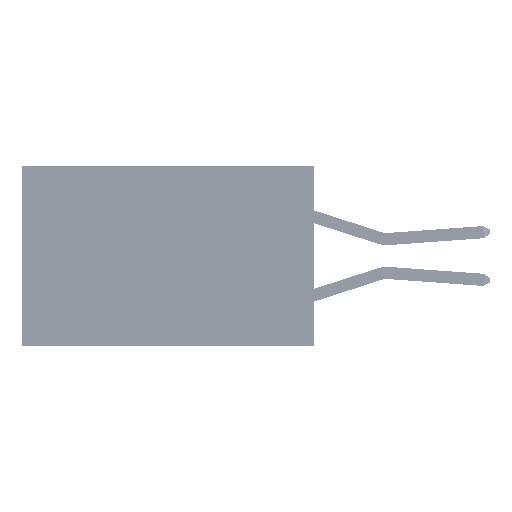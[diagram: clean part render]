
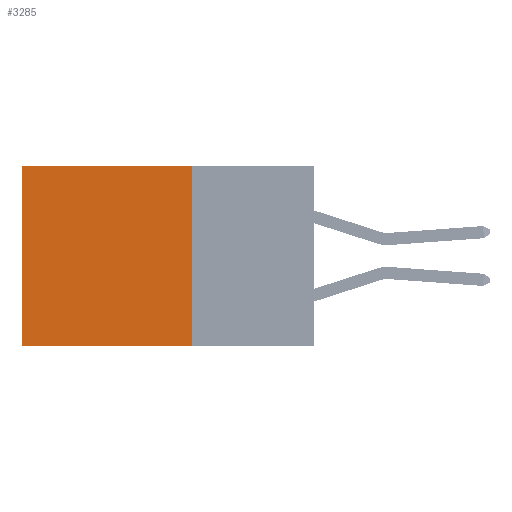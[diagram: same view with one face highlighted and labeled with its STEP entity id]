
A CAD part, left-side view. The second image highlights one B-rep face of the part: STEP entity #3285.
In plain terms, the highlighted planar face has unit normal (-1, 0, 0).
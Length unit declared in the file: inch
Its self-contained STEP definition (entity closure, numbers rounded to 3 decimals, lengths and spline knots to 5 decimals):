
#3029 = DIRECTION ( 'NONE',  ( 0., 0., -1. ) ) ;
#3264 = DIRECTION ( 'NONE',  ( 0., 0., -1. ) ) ;
#3285 = ADVANCED_FACE ( 'NONE', ( #26537 ), #45594, .F. ) ;
#4082 = CARTESIAN_POINT ( 'NONE',  ( 0.2875, 0.6, 0. ) ) ;
#5097 = EDGE_LOOP ( 'NONE', ( #41890, #22316, #21248, #32112 ) ) ;
#6092 = LINE ( 'NONE', #32702, #40562 ) ;
#8601 = EDGE_CURVE ( 'NONE', #42347, #35411, #6092, .T. ) ;
#11349 = EDGE_CURVE ( 'NONE', #30281, #12257, #35997, .T. ) ;
#12257 = VERTEX_POINT ( 'NONE', #42336 ) ;
#12321 = DIRECTION ( 'NONE',  ( 0., 1., 0. ) ) ;
#15935 = VECTOR ( 'NONE', #3029, 39.37008 ) ;
#16419 = EDGE_CURVE ( 'NONE', #42347, #30281, #29291, .T. ) ;
#17265 = DIRECTION ( 'NONE',  ( 1., 0., 0. ) ) ;
#18096 = DIRECTION ( 'NONE',  ( 0., 1., 0. ) ) ;
#20285 = LINE ( 'NONE', #43575, #38691 ) ;
#21248 = ORIENTED_EDGE ( 'NONE', *, *, #8601, .F. ) ;
#22316 = ORIENTED_EDGE ( 'NONE', *, *, #27021, .F. ) ;
#25839 = AXIS2_PLACEMENT_3D ( 'NONE', #35321, #17265, #3264 ) ;
#26537 = FACE_OUTER_BOUND ( 'NONE', #5097, .T. ) ;
#27021 = EDGE_CURVE ( 'NONE', #35411, #12257, #20285, .T. ) ;
#29291 = LINE ( 'NONE', #40447, #41547 ) ;
#30281 = VERTEX_POINT ( 'NONE', #4082 ) ;
#32112 = ORIENTED_EDGE ( 'NONE', *, *, #16419, .T. ) ;
#32702 = CARTESIAN_POINT ( 'NONE',  ( 0.2875, 0.25, 0. ) ) ;
#35058 = CARTESIAN_POINT ( 'NONE',  ( 0.2875, 0.6, 0. ) ) ;
#35321 = CARTESIAN_POINT ( 'NONE',  ( 0.2875, 0.25, 0. ) ) ;
#35411 = VERTEX_POINT ( 'NONE', #44801 ) ;
#35997 = LINE ( 'NONE', #35058, #15935 ) ;
#37927 = CARTESIAN_POINT ( 'NONE',  ( 0.2875, 0.25, 0. ) ) ;
#38688 = DIRECTION ( 'NONE',  ( 0., 0., -1. ) ) ;
#38691 = VECTOR ( 'NONE', #18096, 39.37008 ) ;
#40447 = CARTESIAN_POINT ( 'NONE',  ( 0.2875, 0.25, 0. ) ) ;
#40562 = VECTOR ( 'NONE', #38688, 39.37008 ) ;
#41547 = VECTOR ( 'NONE', #12321, 39.37008 ) ;
#41890 = ORIENTED_EDGE ( 'NONE', *, *, #11349, .T. ) ;
#42336 = CARTESIAN_POINT ( 'NONE',  ( 0.2875, 0.6, -0.37 ) ) ;
#42347 = VERTEX_POINT ( 'NONE', #37927 ) ;
#43575 = CARTESIAN_POINT ( 'NONE',  ( 0.2875, 0.25, -0.37 ) ) ;
#44801 = CARTESIAN_POINT ( 'NONE',  ( 0.2875, 0.25, -0.37 ) ) ;
#45594 = PLANE ( 'NONE',  #25839 ) ;
